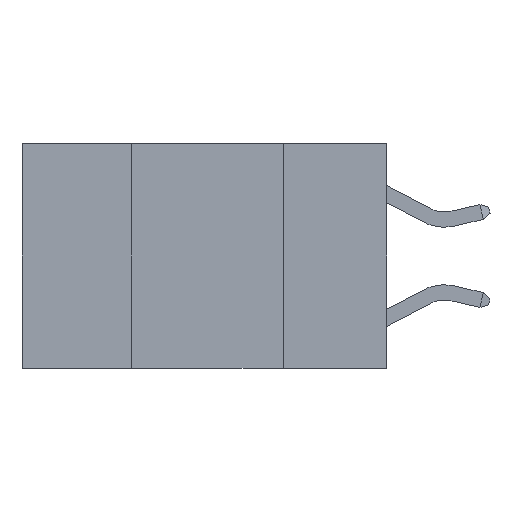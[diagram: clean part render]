
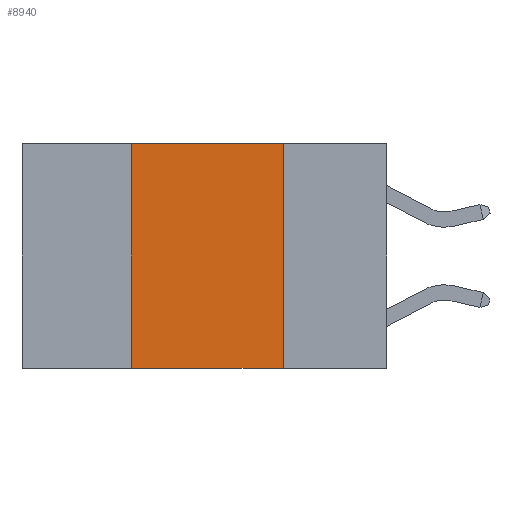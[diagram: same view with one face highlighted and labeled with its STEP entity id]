
A CAD part, left-side view. The second image highlights one B-rep face of the part: STEP entity #8940.
In plain terms, the highlighted planar face has unit normal (-1, 0, 0).
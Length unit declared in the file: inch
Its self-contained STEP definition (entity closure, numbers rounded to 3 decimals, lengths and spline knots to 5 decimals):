
#802 = EDGE_CURVE ( 'NONE', #15709, #1337, #15713, .T. ) ;
#1337 = VERTEX_POINT ( 'NONE', #3018 ) ;
#1621 = DIRECTION ( 'NONE',  ( 1., 0., 0. ) ) ;
#2628 = ORIENTED_EDGE ( 'NONE', *, *, #9471, .F. ) ;
#2671 = VECTOR ( 'NONE', #6521, 39.37008 ) ;
#3018 = CARTESIAN_POINT ( 'NONE',  ( 0., 0.17, 0. ) ) ;
#3773 = CARTESIAN_POINT ( 'NONE',  ( 0., 0.42, 0. ) ) ;
#4818 = EDGE_LOOP ( 'NONE', ( #2628, #8135, #16223, #16175 ) ) ;
#5365 = VERTEX_POINT ( 'NONE', #10302 ) ;
#5598 = DIRECTION ( 'NONE',  ( 0., 0., -1. ) ) ;
#5798 = PLANE ( 'NONE',  #14955 ) ;
#6088 = CARTESIAN_POINT ( 'NONE',  ( 0., 0.6, 0. ) ) ;
#6391 = FACE_OUTER_BOUND ( 'NONE', #4818, .T. ) ;
#6521 = DIRECTION ( 'NONE',  ( 0., 0., 1. ) ) ;
#6829 = LINE ( 'NONE', #3773, #2671 ) ;
#7454 = LINE ( 'NONE', #11163, #10744 ) ;
#8135 = ORIENTED_EDGE ( 'NONE', *, *, #802, .F. ) ;
#8749 = CARTESIAN_POINT ( 'NONE',  ( 0., 0.17, -0.37 ) ) ;
#8940 = ADVANCED_FACE ( 'NONE', ( #6391 ), #5798, .F. ) ;
#9346 = EDGE_CURVE ( 'NONE', #5365, #13744, #9652, .T. ) ;
#9471 = EDGE_CURVE ( 'NONE', #1337, #13744, #7454, .T. ) ;
#9652 = LINE ( 'NONE', #15139, #17080 ) ;
#10014 = CARTESIAN_POINT ( 'NONE',  ( 0., 0.6, 0. ) ) ;
#10302 = CARTESIAN_POINT ( 'NONE',  ( 0., 0.42, -0.37 ) ) ;
#10744 = VECTOR ( 'NONE', #5598, 39.37008 ) ;
#11163 = CARTESIAN_POINT ( 'NONE',  ( 0., 0.17, 0. ) ) ;
#11422 = DIRECTION ( 'NONE',  ( 0., 0., -1. ) ) ;
#12459 = VECTOR ( 'NONE', #15871, 39.37008 ) ;
#13723 = DIRECTION ( 'NONE',  ( 0., -1., 0. ) ) ;
#13744 = VERTEX_POINT ( 'NONE', #8749 ) ;
#14955 = AXIS2_PLACEMENT_3D ( 'NONE', #10014, #1621, #11422 ) ;
#15139 = CARTESIAN_POINT ( 'NONE',  ( 0., 0.6, -0.37 ) ) ;
#15709 = VERTEX_POINT ( 'NONE', #17326 ) ;
#15713 = LINE ( 'NONE', #6088, #12459 ) ;
#15871 = DIRECTION ( 'NONE',  ( 0., -1., 0. ) ) ;
#16175 = ORIENTED_EDGE ( 'NONE', *, *, #9346, .T. ) ;
#16223 = ORIENTED_EDGE ( 'NONE', *, *, #17180, .F. ) ;
#17080 = VECTOR ( 'NONE', #13723, 39.37008 ) ;
#17180 = EDGE_CURVE ( 'NONE', #5365, #15709, #6829, .T. ) ;
#17326 = CARTESIAN_POINT ( 'NONE',  ( 0., 0.42, 0. ) ) ;
